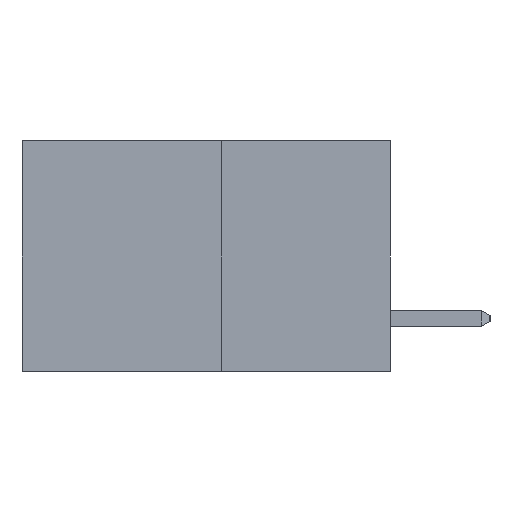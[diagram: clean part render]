
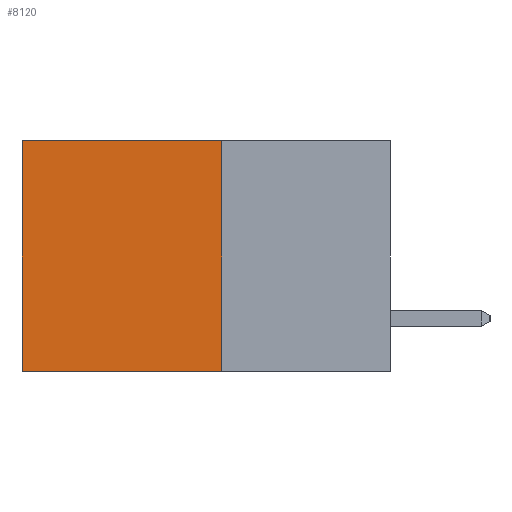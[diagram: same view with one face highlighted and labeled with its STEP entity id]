
A CAD part, left-side view. The second image highlights one B-rep face of the part: STEP entity #8120.
In plain terms, the highlighted planar face has unit normal (-1, 0, 0).
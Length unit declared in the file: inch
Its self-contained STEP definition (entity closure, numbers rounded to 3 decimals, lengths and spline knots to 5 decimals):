
#152 = DIRECTION ( 'NONE',  ( 0., 1., 0. ) ) ;
#164 = LINE ( 'NONE', #5473, #17617 ) ;
#231 = CARTESIAN_POINT ( 'NONE',  ( 0.277, 0.27, -0.37 ) ) ;
#264 = VERTEX_POINT ( 'NONE', #10979 ) ;
#1271 = VECTOR ( 'NONE', #152, 39.37008 ) ;
#1349 = CARTESIAN_POINT ( 'NONE',  ( 0.277, 0.59, -0.37 ) ) ;
#1514 = CARTESIAN_POINT ( 'NONE',  ( 0.277, 0.27, -0.37 ) ) ;
#1845 = CARTESIAN_POINT ( 'NONE',  ( 0.277, 0.27, 0. ) ) ;
#3164 = ORIENTED_EDGE ( 'NONE', *, *, #13937, .T. ) ;
#4316 = DIRECTION ( 'NONE',  ( 0., 1., 0. ) ) ;
#4376 = VECTOR ( 'NONE', #10633, 39.37008 ) ;
#4998 = LINE ( 'NONE', #11187, #1271 ) ;
#5473 = CARTESIAN_POINT ( 'NONE',  ( 0.277, 0.59, -0.37 ) ) ;
#5498 = EDGE_CURVE ( 'NONE', #6629, #16208, #10983, .T. ) ;
#5910 = ORIENTED_EDGE ( 'NONE', *, *, #8840, .F. ) ;
#6629 = VERTEX_POINT ( 'NONE', #1514 ) ;
#7136 = LINE ( 'NONE', #231, #4376 ) ;
#7494 = ORIENTED_EDGE ( 'NONE', *, *, #13823, .T. ) ;
#7651 = ORIENTED_EDGE ( 'NONE', *, *, #5498, .F. ) ;
#8120 = ADVANCED_FACE ( 'NONE', ( #16009 ), #12196, .F. ) ;
#8840 = EDGE_CURVE ( 'NONE', #10413, #6629, #7136, .T. ) ;
#9569 = DIRECTION ( 'NONE',  ( 0., 0., -1. ) ) ;
#10413 = VERTEX_POINT ( 'NONE', #1845 ) ;
#10529 = VECTOR ( 'NONE', #4316, 39.37008 ) ;
#10633 = DIRECTION ( 'NONE',  ( 0., 0., -1. ) ) ;
#10753 = AXIS2_PLACEMENT_3D ( 'NONE', #12302, #12324, #12087 ) ;
#10979 = CARTESIAN_POINT ( 'NONE',  ( 0.277, 0.59, 0. ) ) ;
#10983 = LINE ( 'NONE', #17578, #10529 ) ;
#11187 = CARTESIAN_POINT ( 'NONE',  ( 0.277, 0.27, 0. ) ) ;
#12087 = DIRECTION ( 'NONE',  ( 0., 0., -1. ) ) ;
#12196 = PLANE ( 'NONE',  #10753 ) ;
#12302 = CARTESIAN_POINT ( 'NONE',  ( 0.277, 0.27, -0.37 ) ) ;
#12324 = DIRECTION ( 'NONE',  ( 1., 0., 0. ) ) ;
#13823 = EDGE_CURVE ( 'NONE', #264, #16208, #164, .T. ) ;
#13937 = EDGE_CURVE ( 'NONE', #10413, #264, #4998, .T. ) ;
#14872 = EDGE_LOOP ( 'NONE', ( #7494, #7651, #5910, #3164 ) ) ;
#16009 = FACE_OUTER_BOUND ( 'NONE', #14872, .T. ) ;
#16208 = VERTEX_POINT ( 'NONE', #1349 ) ;
#17578 = CARTESIAN_POINT ( 'NONE',  ( 0.277, 0.27, -0.37 ) ) ;
#17617 = VECTOR ( 'NONE', #9569, 39.37008 ) ;
